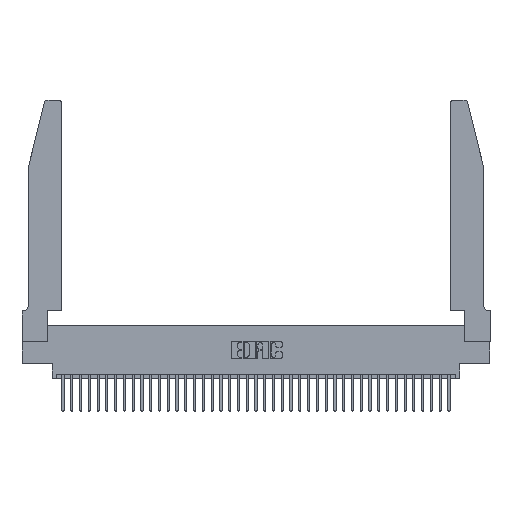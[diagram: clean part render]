
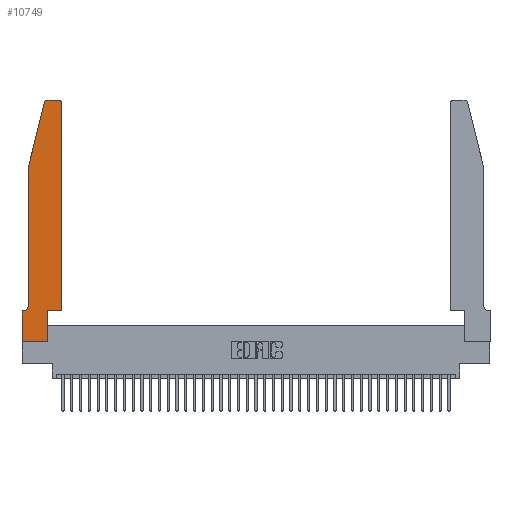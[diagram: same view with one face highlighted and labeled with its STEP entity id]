
A CAD part, top view. The second image highlights one B-rep face of the part: STEP entity #10749.
In plain terms, the highlighted planar face has unit normal (0, 0, 1).
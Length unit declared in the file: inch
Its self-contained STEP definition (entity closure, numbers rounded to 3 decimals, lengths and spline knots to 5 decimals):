
#90 = CARTESIAN_POINT ( 'NONE',  ( 0., 0.35, 0.37 ) ) ;
#1233 = PLANE ( 'NONE',  #36442 ) ;
#1571 = LINE ( 'NONE', #34151, #17141 ) ;
#1604 = CARTESIAN_POINT ( 'NONE',  ( 0.2865, 0.35, 0.37 ) ) ;
#2012 = DIRECTION ( 'NONE',  ( -1., 0., 0. ) ) ;
#2133 = EDGE_CURVE ( 'NONE', #8178, #16576, #11548, .T. ) ;
#2978 = DIRECTION ( 'NONE',  ( 0., 1., 0. ) ) ;
#3247 = CARTESIAN_POINT ( 'NONE',  ( 0.4205, 2.75, 0.37 ) ) ;
#4687 = LINE ( 'NONE', #33559, #34430 ) ;
#4984 = VECTOR ( 'NONE', #11000, 39.37008 ) ;
#5817 = CARTESIAN_POINT ( 'NONE',  ( 0.4505, 0.35, 0.37 ) ) ;
#5994 = CARTESIAN_POINT ( 'NONE',  ( 0.0055, 0.42, 0.37 ) ) ;
#6337 = LINE ( 'NONE', #36776, #21742 ) ;
#6363 = EDGE_CURVE ( 'NONE', #8561, #38045, #39331, .T. ) ;
#6439 = ORIENTED_EDGE ( 'NONE', *, *, #21424, .T. ) ;
#6576 = EDGE_CURVE ( 'NONE', #19640, #8178, #8329, .T. ) ;
#6589 = AXIS2_PLACEMENT_3D ( 'NONE', #9735, #31082, #12782 ) ;
#7224 = LINE ( 'NONE', #8145, #21643 ) ;
#7773 = CARTESIAN_POINT ( 'NONE',  ( 0.25487, 2.72718, 0.37 ) ) ;
#7913 = CARTESIAN_POINT ( 'NONE',  ( 0.0755, 2., 0.37 ) ) ;
#8145 = CARTESIAN_POINT ( 'NONE',  ( 0.0755, 0.35, 0.37 ) ) ;
#8178 = VERTEX_POINT ( 'NONE', #1604 ) ;
#8203 = VERTEX_POINT ( 'NONE', #32465 ) ;
#8329 = LINE ( 'NONE', #24610, #33653 ) ;
#8561 = VERTEX_POINT ( 'NONE', #3247 ) ;
#9150 = DIRECTION ( 'NONE',  ( -1., 0., 0. ) ) ;
#9234 = CARTESIAN_POINT ( 'NONE',  ( 0.0755, 2., 0.37 ) ) ;
#9735 = CARTESIAN_POINT ( 'NONE',  ( 0.4205, 2.72, 0.37 ) ) ;
#9889 = EDGE_CURVE ( 'NONE', #22151, #22782, #31065, .T. ) ;
#10749 = ADVANCED_FACE ( 'NONE', ( #12581 ), #1233, .T. ) ;
#11000 = DIRECTION ( 'NONE',  ( 0., -1., 0. ) ) ;
#11548 = LINE ( 'NONE', #5817, #19695 ) ;
#11595 = CARTESIAN_POINT ( 'NONE',  ( 0.4505, 2.72, 0.37 ) ) ;
#11599 = VERTEX_POINT ( 'NONE', #31984 ) ;
#11969 = EDGE_CURVE ( 'NONE', #18500, #19640, #4687, .T. ) ;
#12581 = FACE_OUTER_BOUND ( 'NONE', #13201, .T. ) ;
#12782 = DIRECTION ( 'NONE',  ( 1., 0., 0. ) ) ;
#12977 = CARTESIAN_POINT ( 'NONE',  ( 0.2865, 0., 0.37 ) ) ;
#13201 = EDGE_LOOP ( 'NONE', ( #31247, #23228, #21604, #27506, #19944, #35123, #17949, #17540, #31947, #38089, #6439, #18155 ) ) ;
#13633 = CARTESIAN_POINT ( 'NONE',  ( 0.0755, 2., 0.37 ) ) ;
#14980 = DIRECTION ( 'NONE',  ( 1., 0., 0. ) ) ;
#15060 = VECTOR ( 'NONE', #2012, 39.37008 ) ;
#15770 = EDGE_CURVE ( 'NONE', #38465, #8561, #25145, .T. ) ;
#16399 = CARTESIAN_POINT ( 'NONE',  ( 0., 0., 0.37 ) ) ;
#16576 = VERTEX_POINT ( 'NONE', #34992 ) ;
#16790 = DIRECTION ( 'NONE',  ( 0., 0., 1. ) ) ;
#16890 = CARTESIAN_POINT ( 'NONE',  ( 0., 0.35, 0.37 ) ) ;
#17141 = VECTOR ( 'NONE', #18989, 39.37008 ) ;
#17514 = CARTESIAN_POINT ( 'NONE',  ( 0.2605, 2.75, 0.37 ) ) ;
#17540 = ORIENTED_EDGE ( 'NONE', *, *, #11969, .T. ) ;
#17949 = ORIENTED_EDGE ( 'NONE', *, *, #34386, .T. ) ;
#18155 = ORIENTED_EDGE ( 'NONE', *, *, #15770, .T. ) ;
#18500 = VERTEX_POINT ( 'NONE', #16399 ) ;
#18989 = DIRECTION ( 'NONE',  ( 0., 1., 0. ) ) ;
#19438 = AXIS2_PLACEMENT_3D ( 'NONE', #5994, #27438, #9150 ) ;
#19640 = VERTEX_POINT ( 'NONE', #12977 ) ;
#19695 = VECTOR ( 'NONE', #14980, 39.37008 ) ;
#19944 = ORIENTED_EDGE ( 'NONE', *, *, #25228, .T. ) ;
#19989 = DIRECTION ( 'NONE',  ( 1., 0., 0. ) ) ;
#21424 = EDGE_CURVE ( 'NONE', #16576, #38465, #1571, .T. ) ;
#21604 = ORIENTED_EDGE ( 'NONE', *, *, #9889, .T. ) ;
#21643 = VECTOR ( 'NONE', #35618, 39.37008 ) ;
#21742 = VECTOR ( 'NONE', #39813, 39.37008 ) ;
#22151 = VERTEX_POINT ( 'NONE', #7773 ) ;
#22165 = EDGE_CURVE ( 'NONE', #22782, #11599, #37531, .T. ) ;
#22782 = VERTEX_POINT ( 'NONE', #13633 ) ;
#23228 = ORIENTED_EDGE ( 'NONE', *, *, #26500, .T. ) ;
#24610 = CARTESIAN_POINT ( 'NONE',  ( 0.2865, 0.35, 0.37 ) ) ;
#25145 = CIRCLE ( 'NONE', #6589, 0.03 ) ;
#25228 = EDGE_CURVE ( 'NONE', #11599, #8203, #32524, .T. ) ;
#26500 = EDGE_CURVE ( 'NONE', #38045, #22151, #28153, .T. ) ;
#27438 = DIRECTION ( 'NONE',  ( 0., 0., -1. ) ) ;
#27506 = ORIENTED_EDGE ( 'NONE', *, *, #22165, .T. ) ;
#28153 = CIRCLE ( 'NONE', #37517, 0.03 ) ;
#29045 = EDGE_CURVE ( 'NONE', #8203, #35223, #7224, .T. ) ;
#30143 = VECTOR ( 'NONE', #36664, 39.37008 ) ;
#31065 = LINE ( 'NONE', #9234, #30143 ) ;
#31082 = DIRECTION ( 'NONE',  ( 0., 0., 1. ) ) ;
#31247 = ORIENTED_EDGE ( 'NONE', *, *, #6363, .T. ) ;
#31947 = ORIENTED_EDGE ( 'NONE', *, *, #6576, .T. ) ;
#31984 = CARTESIAN_POINT ( 'NONE',  ( 0.0755, 0.42, 0.37 ) ) ;
#32465 = CARTESIAN_POINT ( 'NONE',  ( 0.0055, 0.35, 0.37 ) ) ;
#32524 = CIRCLE ( 'NONE', #19438, 0.07 ) ;
#33559 = CARTESIAN_POINT ( 'NONE',  ( 0., 0., 0.37 ) ) ;
#33653 = VECTOR ( 'NONE', #2978, 39.37008 ) ;
#34151 = CARTESIAN_POINT ( 'NONE',  ( 0.4505, 0.35, 0.37 ) ) ;
#34386 = EDGE_CURVE ( 'NONE', #35223, #18500, #6337, .T. ) ;
#34430 = VECTOR ( 'NONE', #36592, 39.37008 ) ;
#34992 = CARTESIAN_POINT ( 'NONE',  ( 0.4505, 0.35, 0.37 ) ) ;
#35048 = CARTESIAN_POINT ( 'NONE',  ( 0.284, 2.72, 0.37 ) ) ;
#35123 = ORIENTED_EDGE ( 'NONE', *, *, #29045, .T. ) ;
#35223 = VERTEX_POINT ( 'NONE', #90 ) ;
#35618 = DIRECTION ( 'NONE',  ( -1., 0., 0. ) ) ;
#36442 = AXIS2_PLACEMENT_3D ( 'NONE', #16890, #38160, #19989 ) ;
#36592 = DIRECTION ( 'NONE',  ( 1., 0., 0. ) ) ;
#36664 = DIRECTION ( 'NONE',  ( -0.239, -0.971, 0. ) ) ;
#36776 = CARTESIAN_POINT ( 'NONE',  ( 0., 0., 0.37 ) ) ;
#37195 = CARTESIAN_POINT ( 'NONE',  ( 0.284, 2.75, 0.37 ) ) ;
#37517 = AXIS2_PLACEMENT_3D ( 'NONE', #35048, #16790, #38063 ) ;
#37531 = LINE ( 'NONE', #7913, #4984 ) ;
#38045 = VERTEX_POINT ( 'NONE', #37195 ) ;
#38063 = DIRECTION ( 'NONE',  ( 1., 0., 0. ) ) ;
#38089 = ORIENTED_EDGE ( 'NONE', *, *, #2133, .T. ) ;
#38160 = DIRECTION ( 'NONE',  ( 0., 0., 1. ) ) ;
#38465 = VERTEX_POINT ( 'NONE', #11595 ) ;
#39331 = LINE ( 'NONE', #17514, #15060 ) ;
#39813 = DIRECTION ( 'NONE',  ( 0., -1., 0. ) ) ;
